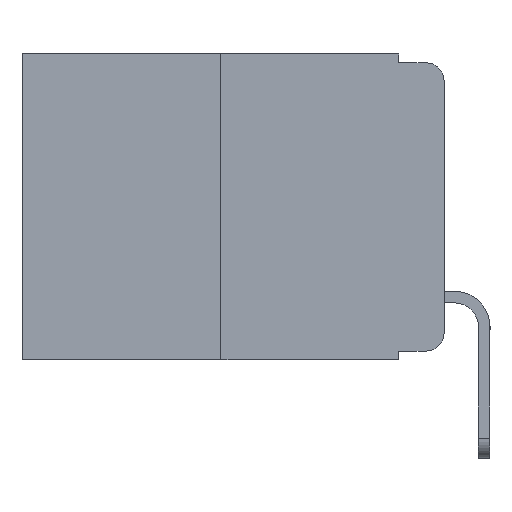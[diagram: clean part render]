
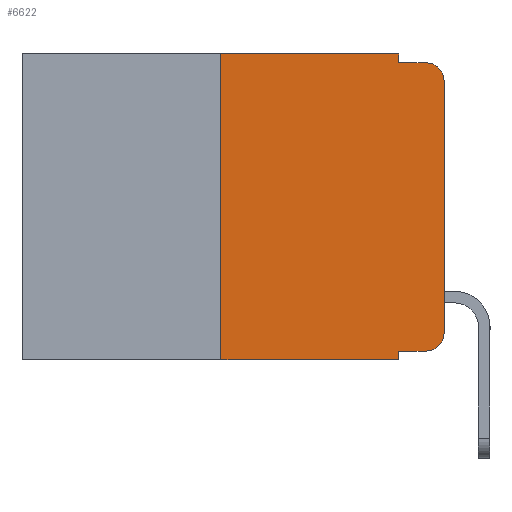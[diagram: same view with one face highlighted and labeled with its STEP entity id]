
A CAD part, left-side view. The second image highlights one B-rep face of the part: STEP entity #6622.
In plain terms, the highlighted planar face has unit normal (-1, 0, 0).
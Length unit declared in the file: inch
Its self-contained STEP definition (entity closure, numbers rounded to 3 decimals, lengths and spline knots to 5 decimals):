
#76 = DIRECTION ( 'NONE',  ( 0., -1., 0. ) ) ;
#288 = ORIENTED_EDGE ( 'NONE', *, *, #4966, .F. ) ;
#308 = VERTEX_POINT ( 'NONE', #9573 ) ;
#417 = CARTESIAN_POINT ( 'NONE',  ( 0., 0.02, -0.03 ) ) ;
#772 = CIRCLE ( 'NONE', #7011, 0.02 ) ;
#998 = ORIENTED_EDGE ( 'NONE', *, *, #10299, .F. ) ;
#1088 = VERTEX_POINT ( 'NONE', #10217 ) ;
#1170 = EDGE_LOOP ( 'NONE', ( #11270, #6221, #9923, #998, #7471, #8652, #7117, #288, #11350, #2830 ) ) ;
#1343 = EDGE_CURVE ( 'NONE', #11536, #10248, #2070, .T. ) ;
#1409 = DIRECTION ( 'NONE',  ( 0., -1., 0. ) ) ;
#1650 = DIRECTION ( 'NONE',  ( 0., 0., -1. ) ) ;
#1671 = LINE ( 'NONE', #2247, #4133 ) ;
#1722 = FACE_OUTER_BOUND ( 'NONE', #1170, .T. ) ;
#1802 = CARTESIAN_POINT ( 'NONE',  ( 0., 0.051, 0. ) ) ;
#1938 = LINE ( 'NONE', #4957, #7088 ) ;
#2070 = LINE ( 'NONE', #6113, #3888 ) ;
#2217 = VECTOR ( 'NONE', #3593, 39.37008 ) ;
#2247 = CARTESIAN_POINT ( 'NONE',  ( 0., 0.051, -0.01 ) ) ;
#2830 = ORIENTED_EDGE ( 'NONE', *, *, #6196, .T. ) ;
#3349 = DIRECTION ( 'NONE',  ( 0., -1., 0. ) ) ;
#3568 = VERTEX_POINT ( 'NONE', #12213 ) ;
#3593 = DIRECTION ( 'NONE',  ( 0., 0., 1. ) ) ;
#3686 = LINE ( 'NONE', #11550, #8291 ) ;
#3888 = VECTOR ( 'NONE', #10215, 39.37008 ) ;
#3891 = CARTESIAN_POINT ( 'NONE',  ( 0., 0., -0.313 ) ) ;
#4133 = VECTOR ( 'NONE', #3349, 39.37008 ) ;
#4243 = VERTEX_POINT ( 'NONE', #11311 ) ;
#4332 = CARTESIAN_POINT ( 'NONE',  ( 0., 0.02, -0.313 ) ) ;
#4362 = VECTOR ( 'NONE', #7579, 39.37008 ) ;
#4568 = AXIS2_PLACEMENT_3D ( 'NONE', #5774, #8446, #7588 ) ;
#4957 = CARTESIAN_POINT ( 'NONE',  ( 0., 0.051, 0. ) ) ;
#4966 = EDGE_CURVE ( 'NONE', #11249, #4243, #6803, .T. ) ;
#5261 = DIRECTION ( 'NONE',  ( 0., 0., -1. ) ) ;
#5542 = EDGE_CURVE ( 'NONE', #11249, #308, #10199, .T. ) ;
#5774 = CARTESIAN_POINT ( 'NONE',  ( 0., 0.473, 0. ) ) ;
#5816 = EDGE_CURVE ( 'NONE', #6898, #4243, #10869, .T. ) ;
#6113 = CARTESIAN_POINT ( 'NONE',  ( 0., 0., 0. ) ) ;
#6196 = EDGE_CURVE ( 'NONE', #308, #11536, #10186, .T. ) ;
#6221 = ORIENTED_EDGE ( 'NONE', *, *, #8575, .T. ) ;
#6239 = VECTOR ( 'NONE', #10023, 39.37008 ) ;
#6364 = CARTESIAN_POINT ( 'NONE',  ( 0., 0.051, -0.333 ) ) ;
#6622 = ADVANCED_FACE ( 'NONE', ( #1722 ), #6683, .F. ) ;
#6683 = PLANE ( 'NONE',  #4568 ) ;
#6803 = LINE ( 'NONE', #1802, #4362 ) ;
#6898 = VERTEX_POINT ( 'NONE', #9666 ) ;
#7011 = AXIS2_PLACEMENT_3D ( 'NONE', #417, #7450, #1650 ) ;
#7088 = VECTOR ( 'NONE', #11122, 39.37008 ) ;
#7117 = ORIENTED_EDGE ( 'NONE', *, *, #5816, .T. ) ;
#7328 = LINE ( 'NONE', #11003, #2217 ) ;
#7450 = DIRECTION ( 'NONE',  ( -1., 0., 0. ) ) ;
#7471 = ORIENTED_EDGE ( 'NONE', *, *, #9228, .F. ) ;
#7579 = DIRECTION ( 'NONE',  ( 0., 0., -1. ) ) ;
#7588 = DIRECTION ( 'NONE',  ( 0., 0., -1. ) ) ;
#7793 = CARTESIAN_POINT ( 'NONE',  ( 0., 0.051, 0. ) ) ;
#7870 = CARTESIAN_POINT ( 'NONE',  ( 0., 0.051, -0.333 ) ) ;
#7990 = EDGE_CURVE ( 'NONE', #6898, #8680, #7328, .T. ) ;
#8291 = VECTOR ( 'NONE', #76, 39.37008 ) ;
#8301 = VERTEX_POINT ( 'NONE', #7793 ) ;
#8446 = DIRECTION ( 'NONE',  ( 1., 0., 0. ) ) ;
#8575 = EDGE_CURVE ( 'NONE', #10248, #1088, #772, .T. ) ;
#8652 = ORIENTED_EDGE ( 'NONE', *, *, #7990, .F. ) ;
#8680 = VERTEX_POINT ( 'NONE', #11847 ) ;
#9228 = EDGE_CURVE ( 'NONE', #8680, #8301, #3686, .T. ) ;
#9573 = CARTESIAN_POINT ( 'NONE',  ( 0., 0.02, -0.333 ) ) ;
#9666 = CARTESIAN_POINT ( 'NONE',  ( 0., 0.25, -0.343 ) ) ;
#9710 = EDGE_CURVE ( 'NONE', #3568, #1088, #1671, .T. ) ;
#9923 = ORIENTED_EDGE ( 'NONE', *, *, #9710, .F. ) ;
#10023 = DIRECTION ( 'NONE',  ( 0., -1., 0. ) ) ;
#10062 = CARTESIAN_POINT ( 'NONE',  ( 0., 0.473, -0.343 ) ) ;
#10164 = CARTESIAN_POINT ( 'NONE',  ( 0., 0., -0.03 ) ) ;
#10186 = CIRCLE ( 'NONE', #12291, 0.02 ) ;
#10199 = LINE ( 'NONE', #6364, #12224 ) ;
#10215 = DIRECTION ( 'NONE',  ( 0., 0., 1. ) ) ;
#10217 = CARTESIAN_POINT ( 'NONE',  ( 0., 0.02, -0.01 ) ) ;
#10248 = VERTEX_POINT ( 'NONE', #10164 ) ;
#10299 = EDGE_CURVE ( 'NONE', #8301, #3568, #1938, .T. ) ;
#10554 = DIRECTION ( 'NONE',  ( -1., 0., 0. ) ) ;
#10869 = LINE ( 'NONE', #10062, #6239 ) ;
#11003 = CARTESIAN_POINT ( 'NONE',  ( 0., 0.25, 0. ) ) ;
#11122 = DIRECTION ( 'NONE',  ( 0., 0., -1. ) ) ;
#11249 = VERTEX_POINT ( 'NONE', #7870 ) ;
#11270 = ORIENTED_EDGE ( 'NONE', *, *, #1343, .T. ) ;
#11311 = CARTESIAN_POINT ( 'NONE',  ( 0., 0.051, -0.343 ) ) ;
#11350 = ORIENTED_EDGE ( 'NONE', *, *, #5542, .T. ) ;
#11536 = VERTEX_POINT ( 'NONE', #3891 ) ;
#11550 = CARTESIAN_POINT ( 'NONE',  ( 0., 0.473, 0. ) ) ;
#11847 = CARTESIAN_POINT ( 'NONE',  ( 0., 0.25, 0. ) ) ;
#12213 = CARTESIAN_POINT ( 'NONE',  ( 0., 0.051, -0.01 ) ) ;
#12224 = VECTOR ( 'NONE', #1409, 39.37008 ) ;
#12291 = AXIS2_PLACEMENT_3D ( 'NONE', #4332, #10554, #5261 ) ;
